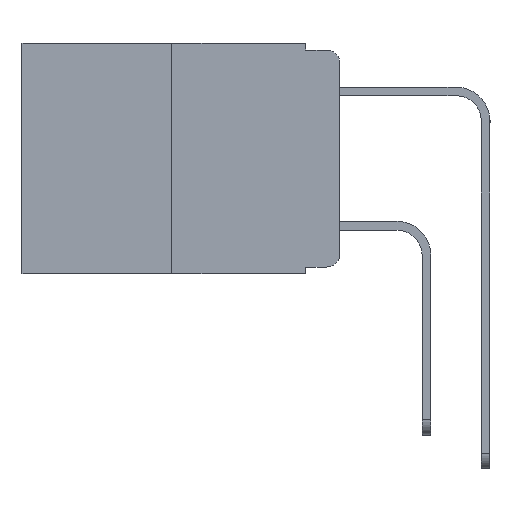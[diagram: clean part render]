
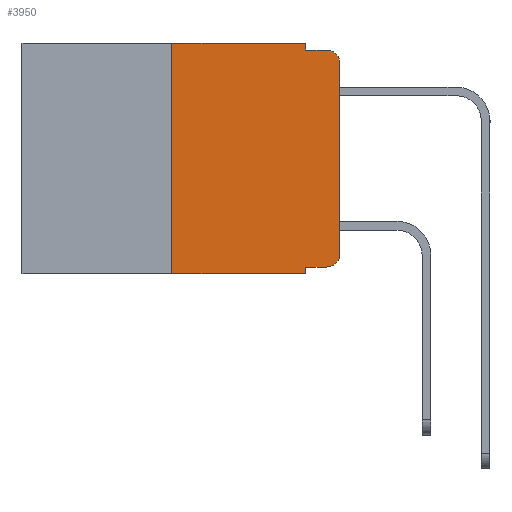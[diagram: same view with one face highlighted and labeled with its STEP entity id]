
A CAD part, left-side view. The second image highlights one B-rep face of the part: STEP entity #3950.
In plain terms, the highlighted planar face has unit normal (-1, 0, 0).
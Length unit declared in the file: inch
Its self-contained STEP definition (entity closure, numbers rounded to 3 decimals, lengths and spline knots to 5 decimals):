
#194 = ORIENTED_EDGE ( 'NONE', *, *, #15817, .T. ) ;
#254 = ORIENTED_EDGE ( 'NONE', *, *, #2595, .F. ) ;
#255 = LINE ( 'NONE', #18197, #13060 ) ;
#849 = DIRECTION ( 'NONE',  ( 0., 0., -1. ) ) ;
#915 = DIRECTION ( 'NONE',  ( 0., -1., 0. ) ) ;
#985 = ORIENTED_EDGE ( 'NONE', *, *, #4904, .F. ) ;
#1386 = CARTESIAN_POINT ( 'NONE',  ( 0., 0.051, 0. ) ) ;
#1796 = VERTEX_POINT ( 'NONE', #11331 ) ;
#1828 = ORIENTED_EDGE ( 'NONE', *, *, #3028, .T. ) ;
#1901 = CIRCLE ( 'NONE', #14230, 0.02 ) ;
#2595 = EDGE_CURVE ( 'NONE', #14193, #6347, #255, .T. ) ;
#2782 = ORIENTED_EDGE ( 'NONE', *, *, #20400, .T. ) ;
#3004 = LINE ( 'NONE', #1386, #19760 ) ;
#3028 = EDGE_CURVE ( 'NONE', #14193, #19235, #10519, .T. ) ;
#3073 = ORIENTED_EDGE ( 'NONE', *, *, #9301, .F. ) ;
#3269 = DIRECTION ( 'NONE',  ( 0., -1., 0. ) ) ;
#3286 = ORIENTED_EDGE ( 'NONE', *, *, #14998, .F. ) ;
#3799 = PLANE ( 'NONE',  #9669 ) ;
#3950 = ADVANCED_FACE ( 'NONE', ( #16639 ), #3799, .F. ) ;
#4077 = DIRECTION ( 'NONE',  ( 0., 0., 1. ) ) ;
#4151 = CARTESIAN_POINT ( 'NONE',  ( 0., 0.02, -0.313 ) ) ;
#4160 = CARTESIAN_POINT ( 'NONE',  ( 0., 0.051, -0.343 ) ) ;
#4366 = ORIENTED_EDGE ( 'NONE', *, *, #10386, .T. ) ;
#4703 = VERTEX_POINT ( 'NONE', #17272 ) ;
#4711 = VERTEX_POINT ( 'NONE', #7602 ) ;
#4904 = EDGE_CURVE ( 'NONE', #7617, #4711, #3004, .T. ) ;
#5151 = VERTEX_POINT ( 'NONE', #11899 ) ;
#5263 = VERTEX_POINT ( 'NONE', #12174 ) ;
#5404 = CARTESIAN_POINT ( 'NONE',  ( 0., 0.25, -0.343 ) ) ;
#5536 = DIRECTION ( 'NONE',  ( 0., 0., -1. ) ) ;
#5869 = DIRECTION ( 'NONE',  ( 0., 0., -1. ) ) ;
#5974 = CARTESIAN_POINT ( 'NONE',  ( 0., 0.02, -0.03 ) ) ;
#6347 = VERTEX_POINT ( 'NONE', #13417 ) ;
#6537 = DIRECTION ( 'NONE',  ( 0., 0., -1. ) ) ;
#6556 = EDGE_LOOP ( 'NONE', ( #12264, #2782, #17853, #985, #3286, #254, #1828, #3073, #4366, #194 ) ) ;
#6743 = VECTOR ( 'NONE', #3269, 39.37008 ) ;
#6933 = DIRECTION ( 'NONE',  ( 0., 0., 1. ) ) ;
#7150 = CARTESIAN_POINT ( 'NONE',  ( 0., 0.473, 0. ) ) ;
#7392 = CARTESIAN_POINT ( 'NONE',  ( 0., 0., 0. ) ) ;
#7602 = CARTESIAN_POINT ( 'NONE',  ( 0., 0.051, -0.01 ) ) ;
#7617 = VERTEX_POINT ( 'NONE', #14466 ) ;
#7633 = DIRECTION ( 'NONE',  ( 0., 0., -1. ) ) ;
#7917 = VECTOR ( 'NONE', #4077, 39.37008 ) ;
#8242 = CARTESIAN_POINT ( 'NONE',  ( 0., 0.473, -0.343 ) ) ;
#8318 = VECTOR ( 'NONE', #849, 39.37008 ) ;
#8402 = LINE ( 'NONE', #7392, #7917 ) ;
#9301 = EDGE_CURVE ( 'NONE', #1796, #19235, #19118, .T. ) ;
#9669 = AXIS2_PLACEMENT_3D ( 'NONE', #7150, #15266, #5536 ) ;
#10084 = CARTESIAN_POINT ( 'NONE',  ( 0., 0.051, -0.01 ) ) ;
#10224 = LINE ( 'NONE', #14119, #17802 ) ;
#10386 = EDGE_CURVE ( 'NONE', #1796, #5151, #18505, .T. ) ;
#10418 = VECTOR ( 'NONE', #19673, 39.37008 ) ;
#10519 = LINE ( 'NONE', #8242, #6743 ) ;
#10784 = EDGE_CURVE ( 'NONE', #4711, #4703, #15238, .T. ) ;
#11331 = CARTESIAN_POINT ( 'NONE',  ( 0., 0.051, -0.333 ) ) ;
#11899 = CARTESIAN_POINT ( 'NONE',  ( 0., 0.02, -0.333 ) ) ;
#12174 = CARTESIAN_POINT ( 'NONE',  ( 0., 0., -0.313 ) ) ;
#12264 = ORIENTED_EDGE ( 'NONE', *, *, #17691, .T. ) ;
#13060 = VECTOR ( 'NONE', #6933, 39.37008 ) ;
#13417 = CARTESIAN_POINT ( 'NONE',  ( 0., 0.25, 0. ) ) ;
#13933 = DIRECTION ( 'NONE',  ( 0., -1., 0. ) ) ;
#14119 = CARTESIAN_POINT ( 'NONE',  ( 0., 0.473, 0. ) ) ;
#14193 = VERTEX_POINT ( 'NONE', #5404 ) ;
#14230 = AXIS2_PLACEMENT_3D ( 'NONE', #4151, #15595, #5869 ) ;
#14253 = VECTOR ( 'NONE', #13933, 39.37008 ) ;
#14466 = CARTESIAN_POINT ( 'NONE',  ( 0., 0.051, 0. ) ) ;
#14998 = EDGE_CURVE ( 'NONE', #6347, #7617, #10224, .T. ) ;
#15238 = LINE ( 'NONE', #10084, #10418 ) ;
#15266 = DIRECTION ( 'NONE',  ( 1., 0., 0. ) ) ;
#15595 = DIRECTION ( 'NONE',  ( -1., 0., 0. ) ) ;
#15607 = CARTESIAN_POINT ( 'NONE',  ( 0., 0.051, 0. ) ) ;
#15817 = EDGE_CURVE ( 'NONE', #5151, #5263, #1901, .T. ) ;
#16639 = FACE_OUTER_BOUND ( 'NONE', #6556, .T. ) ;
#17112 = CARTESIAN_POINT ( 'NONE',  ( 0., 0.051, -0.333 ) ) ;
#17272 = CARTESIAN_POINT ( 'NONE',  ( 0., 0.02, -0.01 ) ) ;
#17306 = DIRECTION ( 'NONE',  ( -1., 0., 0. ) ) ;
#17457 = VERTEX_POINT ( 'NONE', #21141 ) ;
#17691 = EDGE_CURVE ( 'NONE', #5263, #17457, #8402, .T. ) ;
#17802 = VECTOR ( 'NONE', #915, 39.37008 ) ;
#17853 = ORIENTED_EDGE ( 'NONE', *, *, #10784, .F. ) ;
#18197 = CARTESIAN_POINT ( 'NONE',  ( 0., 0.25, 0. ) ) ;
#18505 = LINE ( 'NONE', #17112, #14253 ) ;
#18842 = AXIS2_PLACEMENT_3D ( 'NONE', #5974, #17306, #7633 ) ;
#19118 = LINE ( 'NONE', #15607, #8318 ) ;
#19235 = VERTEX_POINT ( 'NONE', #4160 ) ;
#19673 = DIRECTION ( 'NONE',  ( 0., -1., 0. ) ) ;
#19760 = VECTOR ( 'NONE', #6537, 39.37008 ) ;
#19802 = CIRCLE ( 'NONE', #18842, 0.02 ) ;
#20400 = EDGE_CURVE ( 'NONE', #17457, #4703, #19802, .T. ) ;
#21141 = CARTESIAN_POINT ( 'NONE',  ( 0., 0., -0.03 ) ) ;
